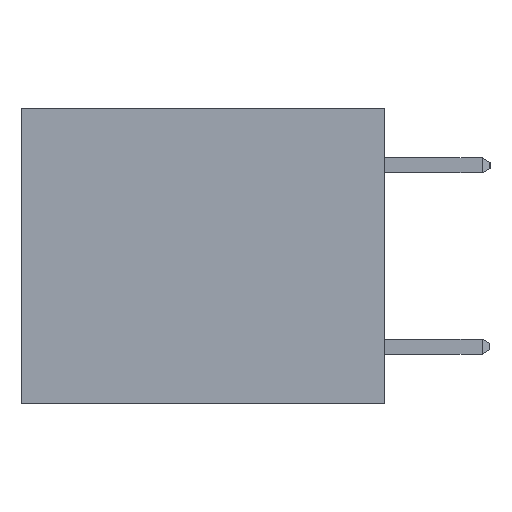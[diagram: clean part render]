
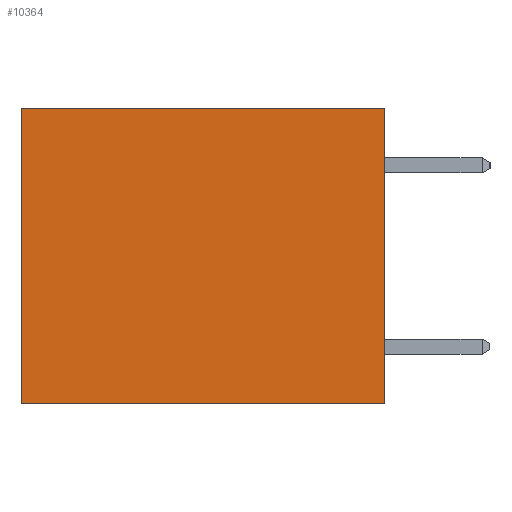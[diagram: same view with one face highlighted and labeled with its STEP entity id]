
A CAD part, left-side view. The second image highlights one B-rep face of the part: STEP entity #10364.
In plain terms, the highlighted planar face has unit normal (-1, 0, 0).
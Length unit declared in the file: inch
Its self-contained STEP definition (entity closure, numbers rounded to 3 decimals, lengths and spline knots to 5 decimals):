
#2152 = LINE ( 'NONE', #17705, #9343 ) ;
#2438 = EDGE_LOOP ( 'NONE', ( #8459, #13424, #15630, #7473 ) ) ;
#2658 = DIRECTION ( 'NONE',  ( 1., 0., 0. ) ) ;
#4646 = CARTESIAN_POINT ( 'NONE',  ( 0.3165, 0.6, 0. ) ) ;
#5471 = EDGE_CURVE ( 'NONE', #7026, #7728, #10068, .T. ) ;
#5793 = DIRECTION ( 'NONE',  ( 0., 0., -1. ) ) ;
#7026 = VERTEX_POINT ( 'NONE', #14978 ) ;
#7473 = ORIENTED_EDGE ( 'NONE', *, *, #13679, .T. ) ;
#7728 = VERTEX_POINT ( 'NONE', #10505 ) ;
#7772 = LINE ( 'NONE', #8957, #14207 ) ;
#8379 = CARTESIAN_POINT ( 'NONE',  ( 0.3165, 0., 0. ) ) ;
#8459 = ORIENTED_EDGE ( 'NONE', *, *, #18018, .T. ) ;
#8957 = CARTESIAN_POINT ( 'NONE',  ( 0.3165, 0., 0. ) ) ;
#9343 = VECTOR ( 'NONE', #5793, 39.37008 ) ;
#9738 = FACE_OUTER_BOUND ( 'NONE', #2438, .T. ) ;
#10068 = LINE ( 'NONE', #18394, #18109 ) ;
#10094 = EDGE_CURVE ( 'NONE', #15289, #7026, #10229, .T. ) ;
#10110 = CARTESIAN_POINT ( 'NONE',  ( 0.3165, 0., -0.49 ) ) ;
#10229 = LINE ( 'NONE', #10927, #14337 ) ;
#10364 = ADVANCED_FACE ( 'NONE', ( #9738 ), #17517, .F. ) ;
#10500 = VERTEX_POINT ( 'NONE', #4646 ) ;
#10505 = CARTESIAN_POINT ( 'NONE',  ( 0.3165, 0.6, -0.49 ) ) ;
#10797 = DIRECTION ( 'NONE',  ( 0., 0., -1. ) ) ;
#10927 = CARTESIAN_POINT ( 'NONE',  ( 0.3165, 0., -0.49 ) ) ;
#11114 = DIRECTION ( 'NONE',  ( 0., 1., 0. ) ) ;
#12394 = AXIS2_PLACEMENT_3D ( 'NONE', #10110, #2658, #12968 ) ;
#12527 = DIRECTION ( 'NONE',  ( 0., 1., 0. ) ) ;
#12968 = DIRECTION ( 'NONE',  ( 0., 0., -1. ) ) ;
#13424 = ORIENTED_EDGE ( 'NONE', *, *, #5471, .F. ) ;
#13679 = EDGE_CURVE ( 'NONE', #15289, #10500, #7772, .T. ) ;
#14207 = VECTOR ( 'NONE', #11114, 39.37008 ) ;
#14337 = VECTOR ( 'NONE', #10797, 39.37008 ) ;
#14978 = CARTESIAN_POINT ( 'NONE',  ( 0.3165, 0., -0.49 ) ) ;
#15289 = VERTEX_POINT ( 'NONE', #8379 ) ;
#15630 = ORIENTED_EDGE ( 'NONE', *, *, #10094, .F. ) ;
#17517 = PLANE ( 'NONE',  #12394 ) ;
#17705 = CARTESIAN_POINT ( 'NONE',  ( 0.3165, 0.6, -0.49 ) ) ;
#18018 = EDGE_CURVE ( 'NONE', #10500, #7728, #2152, .T. ) ;
#18109 = VECTOR ( 'NONE', #12527, 39.37008 ) ;
#18394 = CARTESIAN_POINT ( 'NONE',  ( 0.3165, 0., -0.49 ) ) ;
